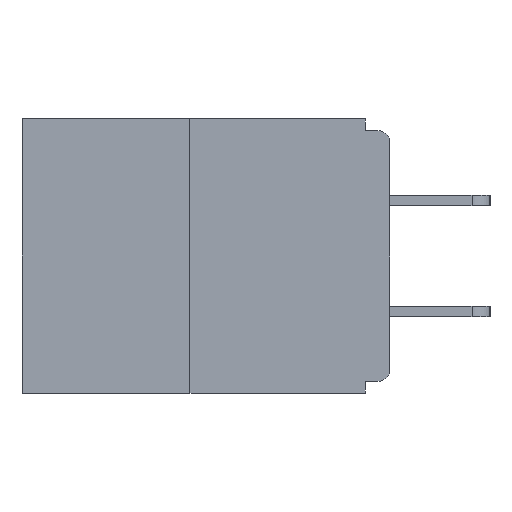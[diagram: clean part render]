
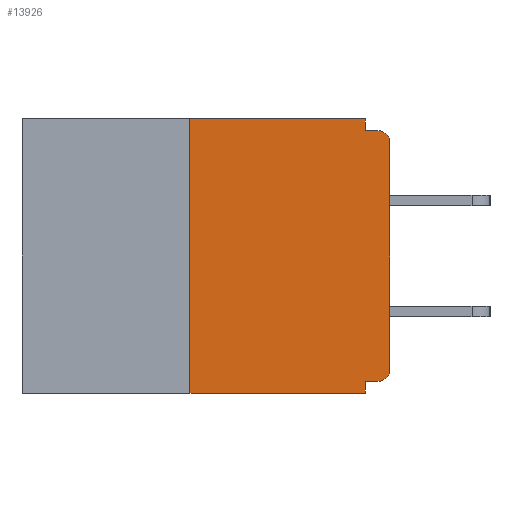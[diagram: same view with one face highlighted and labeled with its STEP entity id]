
A CAD part, left-side view. The second image highlights one B-rep face of the part: STEP entity #13926.
In plain terms, the highlighted planar face has unit normal (-1, 0, 0).
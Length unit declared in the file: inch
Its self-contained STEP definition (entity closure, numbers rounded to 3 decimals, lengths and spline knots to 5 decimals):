
#272 = LINE ( 'NONE', #4487, #8120 ) ;
#287 = AXIS2_PLACEMENT_3D ( 'NONE', #11444, #2640, #12495 ) ;
#527 = VERTEX_POINT ( 'NONE', #2219 ) ;
#686 = VERTEX_POINT ( 'NONE', #11162 ) ;
#790 = DIRECTION ( 'NONE',  ( 0., -1., 0. ) ) ;
#1061 = EDGE_CURVE ( 'NONE', #527, #5103, #272, .T. ) ;
#1468 = CARTESIAN_POINT ( 'NONE',  ( 0., 0.031, -0.015 ) ) ;
#1653 = VERTEX_POINT ( 'NONE', #7759 ) ;
#2088 = DIRECTION ( 'NONE',  ( 0., 0., -1. ) ) ;
#2106 = LINE ( 'NONE', #6005, #11974 ) ;
#2219 = CARTESIAN_POINT ( 'NONE',  ( 0., 0.031, 0. ) ) ;
#2227 = LINE ( 'NONE', #5814, #9537 ) ;
#2255 = EDGE_CURVE ( 'NONE', #5103, #9881, #8082, .T. ) ;
#2285 = CARTESIAN_POINT ( 'NONE',  ( 0., 0.031, -0.343 ) ) ;
#2478 = EDGE_CURVE ( 'NONE', #11266, #686, #11978, .T. ) ;
#2640 = DIRECTION ( 'NONE',  ( 1., 0., 0. ) ) ;
#3029 = VERTEX_POINT ( 'NONE', #8341 ) ;
#3082 = LINE ( 'NONE', #3464, #9061 ) ;
#3239 = DIRECTION ( 'NONE',  ( -1., 0., 0. ) ) ;
#3282 = CARTESIAN_POINT ( 'NONE',  ( 0., 0.031, -0.328 ) ) ;
#3341 = LINE ( 'NONE', #2285, #9302 ) ;
#3464 = CARTESIAN_POINT ( 'NONE',  ( 0., 0.46, 0. ) ) ;
#3517 = CARTESIAN_POINT ( 'NONE',  ( 0., 0., -0.03 ) ) ;
#3630 = CARTESIAN_POINT ( 'NONE',  ( 0., 0.25, -0.343 ) ) ;
#4487 = CARTESIAN_POINT ( 'NONE',  ( 0., 0.031, 0. ) ) ;
#4568 = DIRECTION ( 'NONE',  ( 0., -1., 0. ) ) ;
#4684 = VECTOR ( 'NONE', #10141, 39.37008 ) ;
#4793 = EDGE_CURVE ( 'NONE', #11266, #3029, #2227, .T. ) ;
#5103 = VERTEX_POINT ( 'NONE', #1468 ) ;
#5161 = ORIENTED_EDGE ( 'NONE', *, *, #11354, .T. ) ;
#5191 = CARTESIAN_POINT ( 'NONE',  ( 0., 0.015, -0.015 ) ) ;
#5285 = ORIENTED_EDGE ( 'NONE', *, *, #2255, .F. ) ;
#5551 = EDGE_CURVE ( 'NONE', #9005, #1653, #10373, .T. ) ;
#5792 = CIRCLE ( 'NONE', #10177, 0.015 ) ;
#5814 = CARTESIAN_POINT ( 'NONE',  ( 0., 0.25, 0. ) ) ;
#6005 = CARTESIAN_POINT ( 'NONE',  ( 0., 0., -0.328 ) ) ;
#6309 = CARTESIAN_POINT ( 'NONE',  ( 0., 0.015, -0.313 ) ) ;
#6380 = VECTOR ( 'NONE', #4568, 39.37008 ) ;
#6485 = AXIS2_PLACEMENT_3D ( 'NONE', #6309, #11635, #13793 ) ;
#6811 = DIRECTION ( 'NONE',  ( 0., -1., 0. ) ) ;
#6813 = ORIENTED_EDGE ( 'NONE', *, *, #4793, .F. ) ;
#6901 = DIRECTION ( 'NONE',  ( 0., 0., 1. ) ) ;
#6987 = EDGE_CURVE ( 'NONE', #9252, #686, #3341, .T. ) ;
#7135 = FACE_OUTER_BOUND ( 'NONE', #13480, .T. ) ;
#7417 = CARTESIAN_POINT ( 'NONE',  ( 0., 0.015, -0.03 ) ) ;
#7759 = CARTESIAN_POINT ( 'NONE',  ( 0., 0., -0.313 ) ) ;
#7989 = EDGE_CURVE ( 'NONE', #9005, #9252, #2106, .T. ) ;
#8082 = LINE ( 'NONE', #8466, #13498 ) ;
#8120 = VECTOR ( 'NONE', #8843, 39.37008 ) ;
#8341 = CARTESIAN_POINT ( 'NONE',  ( 0., 0.25, 0. ) ) ;
#8427 = DIRECTION ( 'NONE',  ( 0., 0., -1. ) ) ;
#8466 = CARTESIAN_POINT ( 'NONE',  ( 0., 0., -0.015 ) ) ;
#8671 = ORIENTED_EDGE ( 'NONE', *, *, #2478, .T. ) ;
#8843 = DIRECTION ( 'NONE',  ( 0., 0., -1. ) ) ;
#9005 = VERTEX_POINT ( 'NONE', #10245 ) ;
#9061 = VECTOR ( 'NONE', #6811, 39.37008 ) ;
#9130 = ORIENTED_EDGE ( 'NONE', *, *, #5551, .T. ) ;
#9154 = ORIENTED_EDGE ( 'NONE', *, *, #10088, .F. ) ;
#9252 = VERTEX_POINT ( 'NONE', #3282 ) ;
#9302 = VECTOR ( 'NONE', #8427, 39.37008 ) ;
#9372 = PLANE ( 'NONE',  #287 ) ;
#9471 = ORIENTED_EDGE ( 'NONE', *, *, #1061, .F. ) ;
#9537 = VECTOR ( 'NONE', #6901, 39.37008 ) ;
#9881 = VERTEX_POINT ( 'NONE', #5191 ) ;
#10088 = EDGE_CURVE ( 'NONE', #3029, #527, #3082, .T. ) ;
#10141 = DIRECTION ( 'NONE',  ( 0., 0., 1. ) ) ;
#10177 = AXIS2_PLACEMENT_3D ( 'NONE', #7417, #3239, #2088 ) ;
#10245 = CARTESIAN_POINT ( 'NONE',  ( 0., 0.015, -0.328 ) ) ;
#10373 = CIRCLE ( 'NONE', #6485, 0.015 ) ;
#10401 = ORIENTED_EDGE ( 'NONE', *, *, #6987, .F. ) ;
#10481 = LINE ( 'NONE', #12365, #4684 ) ;
#10570 = VERTEX_POINT ( 'NONE', #3517 ) ;
#10708 = EDGE_CURVE ( 'NONE', #10570, #9881, #5792, .T. ) ;
#11004 = CARTESIAN_POINT ( 'NONE',  ( 0., 0.46, -0.343 ) ) ;
#11162 = CARTESIAN_POINT ( 'NONE',  ( 0., 0.031, -0.343 ) ) ;
#11254 = DIRECTION ( 'NONE',  ( 0., 1., 0. ) ) ;
#11266 = VERTEX_POINT ( 'NONE', #3630 ) ;
#11354 = EDGE_CURVE ( 'NONE', #1653, #10570, #10481, .T. ) ;
#11444 = CARTESIAN_POINT ( 'NONE',  ( 0., 0.46, 0. ) ) ;
#11635 = DIRECTION ( 'NONE',  ( -1., 0., 0. ) ) ;
#11785 = ORIENTED_EDGE ( 'NONE', *, *, #7989, .F. ) ;
#11974 = VECTOR ( 'NONE', #11254, 39.37008 ) ;
#11978 = LINE ( 'NONE', #11004, #6380 ) ;
#12365 = CARTESIAN_POINT ( 'NONE',  ( 0., 0., 0. ) ) ;
#12495 = DIRECTION ( 'NONE',  ( 0., 0., -1. ) ) ;
#13095 = ORIENTED_EDGE ( 'NONE', *, *, #10708, .T. ) ;
#13480 = EDGE_LOOP ( 'NONE', ( #9154, #6813, #8671, #10401, #11785, #9130, #5161, #13095, #5285, #9471 ) ) ;
#13498 = VECTOR ( 'NONE', #790, 39.37008 ) ;
#13793 = DIRECTION ( 'NONE',  ( 0., 0., -1. ) ) ;
#13926 = ADVANCED_FACE ( 'NONE', ( #7135 ), #9372, .F. ) ;
